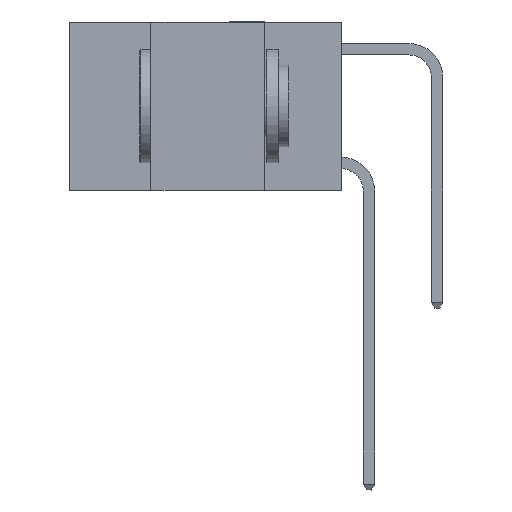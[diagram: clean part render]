
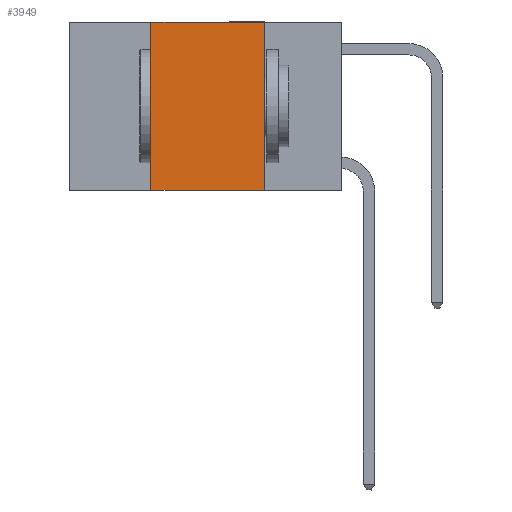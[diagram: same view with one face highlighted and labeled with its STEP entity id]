
A CAD part, left-side view. The second image highlights one B-rep face of the part: STEP entity #3949.
In plain terms, the highlighted planar face has unit normal (-1, 0, 0).
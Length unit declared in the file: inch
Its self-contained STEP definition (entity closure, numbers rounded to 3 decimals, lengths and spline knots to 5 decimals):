
#311 = VERTEX_POINT ( 'NONE', #11027 ) ;
#858 = LINE ( 'NONE', #3538, #9913 ) ;
#1302 = PLANE ( 'NONE',  #1627 ) ;
#1463 = ORIENTED_EDGE ( 'NONE', *, *, #7994, .F. ) ;
#1627 = AXIS2_PLACEMENT_3D ( 'NONE', #4829, #2229, #8383 ) ;
#1822 = CARTESIAN_POINT ( 'NONE',  ( 0., 0.6, -0.37 ) ) ;
#1960 = VERTEX_POINT ( 'NONE', #10533 ) ;
#2229 = DIRECTION ( 'NONE',  ( 1., 0., 0. ) ) ;
#2302 = CARTESIAN_POINT ( 'NONE',  ( 0., 0.6, 0. ) ) ;
#3125 = EDGE_CURVE ( 'NONE', #7545, #1960, #10630, .T. ) ;
#3473 = VECTOR ( 'NONE', #7617, 39.37008 ) ;
#3538 = CARTESIAN_POINT ( 'NONE',  ( 0., 0.42, 0. ) ) ;
#3567 = ORIENTED_EDGE ( 'NONE', *, *, #8832, .T. ) ;
#3949 = ADVANCED_FACE ( 'NONE', ( #4830 ), #1302, .F. ) ;
#4829 = CARTESIAN_POINT ( 'NONE',  ( 0., 0.6, 0. ) ) ;
#4830 = FACE_OUTER_BOUND ( 'NONE', #8809, .T. ) ;
#5317 = CARTESIAN_POINT ( 'NONE',  ( 0., 0.17, 0. ) ) ;
#6181 = ORIENTED_EDGE ( 'NONE', *, *, #3125, .F. ) ;
#6503 = EDGE_CURVE ( 'NONE', #10332, #7545, #10353, .T. ) ;
#7300 = CARTESIAN_POINT ( 'NONE',  ( 0., 0.42, 0. ) ) ;
#7545 = VERTEX_POINT ( 'NONE', #10749 ) ;
#7617 = DIRECTION ( 'NONE',  ( 0., -1., 0. ) ) ;
#7954 = DIRECTION ( 'NONE',  ( 0., 0., -1. ) ) ;
#7994 = EDGE_CURVE ( 'NONE', #311, #10332, #858, .T. ) ;
#8068 = LINE ( 'NONE', #1822, #10043 ) ;
#8135 = VECTOR ( 'NONE', #7954, 39.37008 ) ;
#8383 = DIRECTION ( 'NONE',  ( 0., 0., -1. ) ) ;
#8809 = EDGE_LOOP ( 'NONE', ( #6181, #11126, #1463, #3567 ) ) ;
#8832 = EDGE_CURVE ( 'NONE', #311, #1960, #8068, .T. ) ;
#8847 = DIRECTION ( 'NONE',  ( 0., -1., 0. ) ) ;
#9595 = DIRECTION ( 'NONE',  ( 0., 0., 1. ) ) ;
#9913 = VECTOR ( 'NONE', #9595, 39.37008 ) ;
#10043 = VECTOR ( 'NONE', #8847, 39.37008 ) ;
#10332 = VERTEX_POINT ( 'NONE', #7300 ) ;
#10353 = LINE ( 'NONE', #2302, #3473 ) ;
#10533 = CARTESIAN_POINT ( 'NONE',  ( 0., 0.17, -0.37 ) ) ;
#10630 = LINE ( 'NONE', #5317, #8135 ) ;
#10749 = CARTESIAN_POINT ( 'NONE',  ( 0., 0.17, 0. ) ) ;
#11027 = CARTESIAN_POINT ( 'NONE',  ( 0., 0.42, -0.37 ) ) ;
#11126 = ORIENTED_EDGE ( 'NONE', *, *, #6503, .F. ) ;
